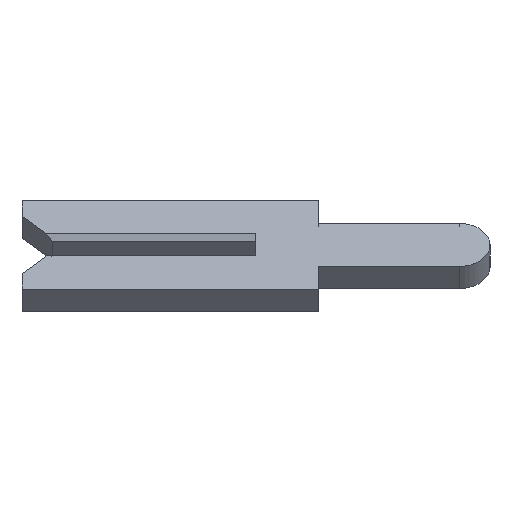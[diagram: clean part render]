
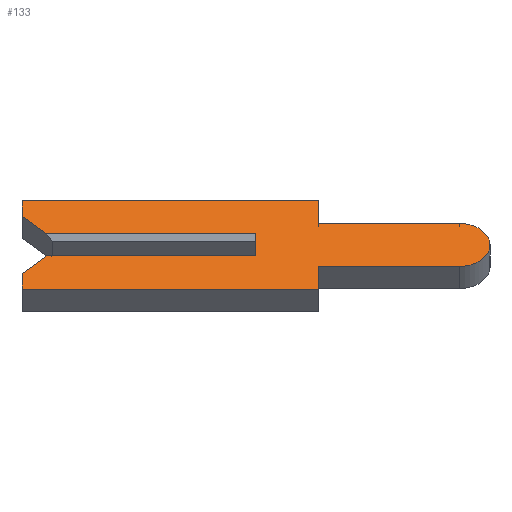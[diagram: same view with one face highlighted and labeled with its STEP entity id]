
A CAD part, left-side view. The second image highlights one B-rep face of the part: STEP entity #133.
In plain terms, the highlighted face is planar.
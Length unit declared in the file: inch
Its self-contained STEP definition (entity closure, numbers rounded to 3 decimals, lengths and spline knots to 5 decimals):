
#2 = DIRECTION ( 'NONE',  ( 0., -1., 0. ) ) ;
#18 = CARTESIAN_POINT ( 'NONE',  ( -0.01, 0.15, 0.026 ) ) ;
#38 = ORIENTED_EDGE ( 'NONE', *, *, #1110, .F. ) ;
#40 = ORIENTED_EDGE ( 'NONE', *, *, #699, .F. ) ;
#53 = CARTESIAN_POINT ( 'NONE',  ( -0.01, 0.1305, -0.0065 ) ) ;
#54 = VECTOR ( 'NONE', #771, 39.37008 ) ;
#63 = ORIENTED_EDGE ( 'NONE', *, *, #632, .F. ) ;
#84 = CARTESIAN_POINT ( 'NONE',  ( -0.01, -0.1305, -0.01 ) ) ;
#88 = EDGE_CURVE ( 'NONE', #1003, #809, #589, .T. ) ;
#91 = CARTESIAN_POINT ( 'NONE',  ( -0.01, 0., 0.01 ) ) ;
#101 = CARTESIAN_POINT ( 'NONE',  ( -0.01, 0.15, 0.026 ) ) ;
#110 = DIRECTION ( 'NONE',  ( 0., 1., 0. ) ) ;
#113 = LINE ( 'NONE', #875, #434 ) ;
#125 = DIRECTION ( 'NONE',  ( 0., 0., -1. ) ) ;
#129 = CARTESIAN_POINT ( 'NONE',  ( -0.01, -0.04, -0.04 ) ) ;
#133 = ADVANCED_FACE ( 'NONE', ( #960 ), #531, .F. ) ;
#138 = VERTEX_POINT ( 'NONE', #538 ) ;
#150 = VERTEX_POINT ( 'NONE', #166 ) ;
#166 = CARTESIAN_POINT ( 'NONE',  ( -0.01, 0.15, -0.026 ) ) ;
#171 = CARTESIAN_POINT ( 'NONE',  ( -0.01, -0.04, 0.0195 ) ) ;
#182 = LINE ( 'NONE', #609, #1034 ) ;
#184 = ORIENTED_EDGE ( 'NONE', *, *, #263, .T. ) ;
#191 = ORIENTED_EDGE ( 'NONE', *, *, #460, .F. ) ;
#203 = ORIENTED_EDGE ( 'NONE', *, *, #601, .F. ) ;
#223 = VERTEX_POINT ( 'NONE', #91 ) ;
#227 = DIRECTION ( 'NONE',  ( 0., -1., 0. ) ) ;
#243 = EDGE_CURVE ( 'NONE', #138, #509, #1113, .T. ) ;
#249 = CARTESIAN_POINT ( 'NONE',  ( -0.01, -0.04, -0.04 ) ) ;
#250 = EDGE_CURVE ( 'NONE', #256, #1067, #1141, .T. ) ;
#253 = ORIENTED_EDGE ( 'NONE', *, *, #583, .F. ) ;
#256 = VERTEX_POINT ( 'NONE', #366 ) ;
#259 = VECTOR ( 'NONE', #854, 39.37008 ) ;
#263 = EDGE_CURVE ( 'NONE', #1144, #223, #571, .T. ) ;
#287 = LINE ( 'NONE', #593, #628 ) ;
#302 = LINE ( 'NONE', #622, #525 ) ;
#322 = CARTESIAN_POINT ( 'NONE',  ( -0.01, -0.04, 0.04 ) ) ;
#333 = VERTEX_POINT ( 'NONE', #18 ) ;
#334 = CARTESIAN_POINT ( 'NONE',  ( -0.01, 0., -0.01 ) ) ;
#350 = CARTESIAN_POINT ( 'NONE',  ( -0.01, -0.1305, 0. ) ) ;
#352 = DIRECTION ( 'NONE',  ( 0., 1., 0. ) ) ;
#358 = ORIENTED_EDGE ( 'NONE', *, *, #250, .F. ) ;
#365 = EDGE_CURVE ( 'NONE', #509, #521, #287, .T. ) ;
#366 = CARTESIAN_POINT ( 'NONE',  ( -0.01, 0.134, -0.01 ) ) ;
#373 = CARTESIAN_POINT ( 'NONE',  ( -0.01, 0.15, 0.01 ) ) ;
#375 = VECTOR ( 'NONE', #1047, 39.37008 ) ;
#377 = VECTOR ( 'NONE', #558, 39.37008 ) ;
#378 = DIRECTION ( 'NONE',  ( 1., 0., 0. ) ) ;
#386 = CARTESIAN_POINT ( 'NONE',  ( -0.01, -0.04, -0.0195 ) ) ;
#406 = ORIENTED_EDGE ( 'NONE', *, *, #365, .F. ) ;
#413 = AXIS2_PLACEMENT_3D ( 'NONE', #648, #378, #573 ) ;
#421 = LINE ( 'NONE', #129, #375 ) ;
#434 = VECTOR ( 'NONE', #227, 39.37008 ) ;
#450 = CARTESIAN_POINT ( 'NONE',  ( -0.01, 0.15, -0.04 ) ) ;
#460 = EDGE_CURVE ( 'NONE', #809, #150, #994, .T. ) ;
#476 = ORIENTED_EDGE ( 'NONE', *, *, #1140, .F. ) ;
#509 = VERTEX_POINT ( 'NONE', #955 ) ;
#521 = VERTEX_POINT ( 'NONE', #386 ) ;
#525 = VECTOR ( 'NONE', #988, 39.37008 ) ;
#526 = VECTOR ( 'NONE', #2, 39.37008 ) ;
#531 = PLANE ( 'NONE',  #1163 ) ;
#538 = CARTESIAN_POINT ( 'NONE',  ( -0.01, -0.1305, 0.0195 ) ) ;
#552 = VECTOR ( 'NONE', #1138, 39.37008 ) ;
#558 = DIRECTION ( 'NONE',  ( 0., -1., 0. ) ) ;
#571 = LINE ( 'NONE', #373, #377 ) ;
#573 = DIRECTION ( 'NONE',  ( 0., 0., -1. ) ) ;
#580 = CARTESIAN_POINT ( 'NONE',  ( -0.01, 0.15, -0.026 ) ) ;
#583 = EDGE_CURVE ( 'NONE', #1144, #333, #822, .T. ) ;
#589 = LINE ( 'NONE', #450, #927 ) ;
#593 = CARTESIAN_POINT ( 'NONE',  ( -0.01, -0.04, -0.0195 ) ) ;
#601 = EDGE_CURVE ( 'NONE', #333, #788, #753, .T. ) ;
#602 = VERTEX_POINT ( 'NONE', #322 ) ;
#609 = CARTESIAN_POINT ( 'NONE',  ( -0.01, 0., 0.0065 ) ) ;
#617 = CARTESIAN_POINT ( 'NONE',  ( -0.01, 0.134, 0.01 ) ) ;
#618 = EDGE_LOOP ( 'NONE', ( #184, #991, #358, #38, #191, #776, #40, #406, #883, #63, #941, #476, #203, #253 ) ) ;
#622 = CARTESIAN_POINT ( 'NONE',  ( -0.01, 0.15, 0.04 ) ) ;
#628 = VECTOR ( 'NONE', #110, 39.37008 ) ;
#632 = EDGE_CURVE ( 'NONE', #1073, #138, #113, .T. ) ;
#648 = CARTESIAN_POINT ( 'NONE',  ( -0.01, -0.1305, 0. ) ) ;
#675 = CARTESIAN_POINT ( 'NONE',  ( -0.01, 0.1305, 0.0065 ) ) ;
#680 = VECTOR ( 'NONE', #1072, 39.37008 ) ;
#690 = CARTESIAN_POINT ( 'NONE',  ( -0.01, 0.15, 0.04 ) ) ;
#699 = EDGE_CURVE ( 'NONE', #521, #1003, #421, .T. ) ;
#715 = EDGE_CURVE ( 'NONE', #602, #1073, #722, .T. ) ;
#722 = LINE ( 'NONE', #1062, #872 ) ;
#753 = LINE ( 'NONE', #101, #54 ) ;
#768 = EDGE_CURVE ( 'NONE', #1067, #223, #182, .T. ) ;
#771 = DIRECTION ( 'NONE',  ( 0., 0., 1. ) ) ;
#776 = ORIENTED_EDGE ( 'NONE', *, *, #88, .F. ) ;
#788 = VERTEX_POINT ( 'NONE', #690 ) ;
#791 = LINE ( 'NONE', #53, #680 ) ;
#809 = VERTEX_POINT ( 'NONE', #961 ) ;
#822 = LINE ( 'NONE', #675, #552 ) ;
#854 = DIRECTION ( 'NONE',  ( 0., 0., 1. ) ) ;
#872 = VECTOR ( 'NONE', #125, 39.37008 ) ;
#875 = CARTESIAN_POINT ( 'NONE',  ( -0.01, -0.04, 0.0195 ) ) ;
#883 = ORIENTED_EDGE ( 'NONE', *, *, #243, .F. ) ;
#927 = VECTOR ( 'NONE', #352, 39.37008 ) ;
#941 = ORIENTED_EDGE ( 'NONE', *, *, #715, .F. ) ;
#955 = CARTESIAN_POINT ( 'NONE',  ( -0.01, -0.1305, -0.0195 ) ) ;
#960 = FACE_OUTER_BOUND ( 'NONE', #618, .T. ) ;
#961 = CARTESIAN_POINT ( 'NONE',  ( -0.01, 0.15, -0.04 ) ) ;
#964 = DIRECTION ( 'NONE',  ( 0., 0., 1. ) ) ;
#988 = DIRECTION ( 'NONE',  ( 0., -1., 0. ) ) ;
#991 = ORIENTED_EDGE ( 'NONE', *, *, #768, .F. ) ;
#994 = LINE ( 'NONE', #580, #259 ) ;
#1003 = VERTEX_POINT ( 'NONE', #249 ) ;
#1034 = VECTOR ( 'NONE', #964, 39.37008 ) ;
#1047 = DIRECTION ( 'NONE',  ( 0., 0., -1. ) ) ;
#1062 = CARTESIAN_POINT ( 'NONE',  ( -0.01, -0.04, 0.04 ) ) ;
#1067 = VERTEX_POINT ( 'NONE', #334 ) ;
#1072 = DIRECTION ( 'NONE',  ( 0., -0.707, 0.707 ) ) ;
#1073 = VERTEX_POINT ( 'NONE', #171 ) ;
#1097 = DIRECTION ( 'NONE',  ( 1., 0., 0. ) ) ;
#1110 = EDGE_CURVE ( 'NONE', #150, #256, #791, .T. ) ;
#1113 = CIRCLE ( 'NONE', #413, 0.0195 ) ;
#1138 = DIRECTION ( 'NONE',  ( 0., 0.707, 0.707 ) ) ;
#1140 = EDGE_CURVE ( 'NONE', #788, #602, #302, .T. ) ;
#1141 = LINE ( 'NONE', #84, #526 ) ;
#1144 = VERTEX_POINT ( 'NONE', #617 ) ;
#1163 = AXIS2_PLACEMENT_3D ( 'NONE', #350, #1097, #1178 ) ;
#1178 = DIRECTION ( 'NONE',  ( 0., 0., -1. ) ) ;
